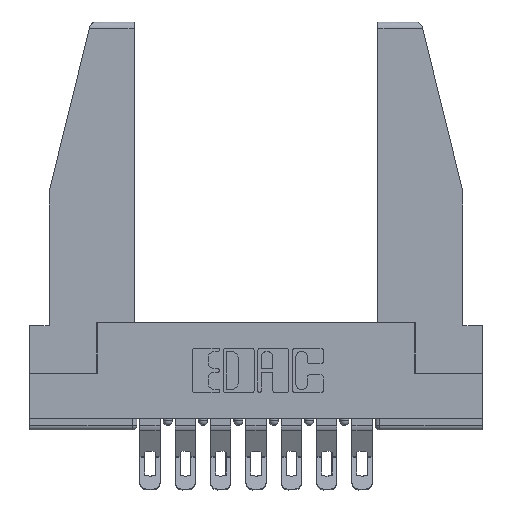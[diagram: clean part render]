
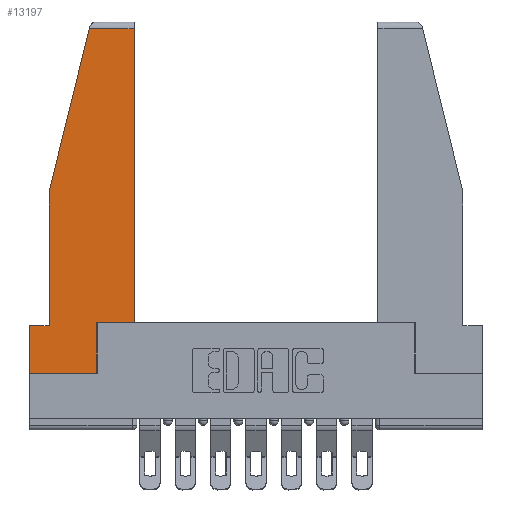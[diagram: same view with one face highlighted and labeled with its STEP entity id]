
A CAD part, top view. The second image highlights one B-rep face of the part: STEP entity #13197.
In plain terms, the highlighted planar face has unit normal (0, 0, 1).
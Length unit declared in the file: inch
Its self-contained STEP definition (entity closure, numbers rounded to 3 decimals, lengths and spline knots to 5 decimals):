
#90 = VERTEX_POINT ( 'NONE', #495 ) ;
#117 = CARTESIAN_POINT ( 'NONE',  ( 0.086, 0.21, 0. ) ) ;
#325 = LINE ( 'NONE', #3770, #1312 ) ;
#362 = CARTESIAN_POINT ( 'NONE',  ( 0.297, 0.223, 0. ) ) ;
#422 = EDGE_LOOP ( 'NONE', ( #8226, #6201, #9857, #6817, #12835, #5437, #7567, #5539, #12540 ) ) ;
#495 = CARTESIAN_POINT ( 'NONE',  ( 0., 0.21, 0. ) ) ;
#520 = CARTESIAN_POINT ( 'NONE',  ( 0., 0.21, 0. ) ) ;
#889 = VECTOR ( 'NONE', #11990, 39.37008 ) ;
#1147 = CARTESIAN_POINT ( 'NONE',  ( 0., 1.52, 0. ) ) ;
#1178 = CARTESIAN_POINT ( 'NONE',  ( 0.297, 0.223, 0. ) ) ;
#1312 = VECTOR ( 'NONE', #1547, 39.37008 ) ;
#1526 = VERTEX_POINT ( 'NONE', #117 ) ;
#1547 = DIRECTION ( 'NONE',  ( -0.239, -0.971, 0. ) ) ;
#1592 = CARTESIAN_POINT ( 'NONE',  ( 0., 0., 0. ) ) ;
#1813 = VECTOR ( 'NONE', #8463, 39.37008 ) ;
#1861 = CARTESIAN_POINT ( 'NONE',  ( 0., 0., 0. ) ) ;
#1999 = EDGE_CURVE ( 'NONE', #7309, #3363, #325, .T. ) ;
#2274 = CARTESIAN_POINT ( 'NONE',  ( 0.086, 0.8, 0. ) ) ;
#2458 = DIRECTION ( 'NONE',  ( 0., 1., 0. ) ) ;
#2644 = DIRECTION ( 'NONE',  ( 0., -1., 0. ) ) ;
#3349 = LINE ( 'NONE', #362, #6146 ) ;
#3363 = VERTEX_POINT ( 'NONE', #2274 ) ;
#3601 = CARTESIAN_POINT ( 'NONE',  ( 0.461, 0.223, 0. ) ) ;
#3629 = DIRECTION ( 'NONE',  ( 1., 0., 0. ) ) ;
#3770 = CARTESIAN_POINT ( 'NONE',  ( 0.271, 1.55, 0. ) ) ;
#3866 = VECTOR ( 'NONE', #2458, 39.37008 ) ;
#3946 = LINE ( 'NONE', #1147, #1813 ) ;
#4187 = EDGE_CURVE ( 'NONE', #5553, #9948, #3349, .T. ) ;
#4258 = DIRECTION ( 'NONE',  ( 1., 0., 0. ) ) ;
#4366 = CARTESIAN_POINT ( 'NONE',  ( 0.2636, 1.52, 0. ) ) ;
#4369 = CARTESIAN_POINT ( 'NONE',  ( 0.461, 0.223, 0. ) ) ;
#4576 = CARTESIAN_POINT ( 'NONE',  ( 0.461, 1.52, 0. ) ) ;
#4692 = DIRECTION ( 'NONE',  ( -1., 0., 0. ) ) ;
#4733 = CARTESIAN_POINT ( 'NONE',  ( 0., 0.21, 0. ) ) ;
#4796 = CARTESIAN_POINT ( 'NONE',  ( 0., 0., 0. ) ) ;
#4807 = VERTEX_POINT ( 'NONE', #4576 ) ;
#4855 = CARTESIAN_POINT ( 'NONE',  ( 0.297, 0., 0. ) ) ;
#5427 = AXIS2_PLACEMENT_3D ( 'NONE', #1861, #13531, #4258 ) ;
#5437 = ORIENTED_EDGE ( 'NONE', *, *, #6322, .T. ) ;
#5539 = ORIENTED_EDGE ( 'NONE', *, *, #10140, .T. ) ;
#5553 = VERTEX_POINT ( 'NONE', #1178 ) ;
#5555 = CARTESIAN_POINT ( 'NONE',  ( 0.297, 0., 0. ) ) ;
#5846 = LINE ( 'NONE', #3601, #3866 ) ;
#6127 = LINE ( 'NONE', #7533, #7587 ) ;
#6146 = VECTOR ( 'NONE', #3629, 39.37008 ) ;
#6201 = ORIENTED_EDGE ( 'NONE', *, *, #6682, .T. ) ;
#6322 = EDGE_CURVE ( 'NONE', #90, #11217, #8530, .T. ) ;
#6682 = EDGE_CURVE ( 'NONE', #4807, #7309, #3946, .T. ) ;
#6817 = ORIENTED_EDGE ( 'NONE', *, *, #12252, .T. ) ;
#7309 = VERTEX_POINT ( 'NONE', #4366 ) ;
#7518 = VECTOR ( 'NONE', #4692, 39.37008 ) ;
#7533 = CARTESIAN_POINT ( 'NONE',  ( 0.086, 0.8, 0. ) ) ;
#7567 = ORIENTED_EDGE ( 'NONE', *, *, #10977, .T. ) ;
#7587 = VECTOR ( 'NONE', #8563, 39.37008 ) ;
#8046 = EDGE_CURVE ( 'NONE', #1526, #90, #10918, .T. ) ;
#8186 = PLANE ( 'NONE',  #5427 ) ;
#8205 = FACE_OUTER_BOUND ( 'NONE', #422, .T. ) ;
#8226 = ORIENTED_EDGE ( 'NONE', *, *, #10840, .T. ) ;
#8463 = DIRECTION ( 'NONE',  ( -1., 0., 0. ) ) ;
#8530 = LINE ( 'NONE', #520, #13094 ) ;
#8563 = DIRECTION ( 'NONE',  ( 0., -1., 0. ) ) ;
#8775 = DIRECTION ( 'NONE',  ( 0., 1., 0. ) ) ;
#9252 = LINE ( 'NONE', #4796, #889 ) ;
#9439 = LINE ( 'NONE', #5555, #11381 ) ;
#9857 = ORIENTED_EDGE ( 'NONE', *, *, #1999, .T. ) ;
#9948 = VERTEX_POINT ( 'NONE', #4369 ) ;
#10140 = EDGE_CURVE ( 'NONE', #11886, #5553, #9439, .T. ) ;
#10840 = EDGE_CURVE ( 'NONE', #9948, #4807, #5846, .T. ) ;
#10918 = LINE ( 'NONE', #4733, #7518 ) ;
#10977 = EDGE_CURVE ( 'NONE', #11217, #11886, #9252, .T. ) ;
#11217 = VERTEX_POINT ( 'NONE', #1592 ) ;
#11381 = VECTOR ( 'NONE', #8775, 39.37008 ) ;
#11886 = VERTEX_POINT ( 'NONE', #4855 ) ;
#11990 = DIRECTION ( 'NONE',  ( 1., 0., 0. ) ) ;
#12252 = EDGE_CURVE ( 'NONE', #3363, #1526, #6127, .T. ) ;
#12540 = ORIENTED_EDGE ( 'NONE', *, *, #4187, .T. ) ;
#12835 = ORIENTED_EDGE ( 'NONE', *, *, #8046, .T. ) ;
#13094 = VECTOR ( 'NONE', #2644, 39.37008 ) ;
#13197 = ADVANCED_FACE ( 'NONE', ( #8205 ), #8186, .T. ) ;
#13531 = DIRECTION ( 'NONE',  ( 0., 0., 1. ) ) ;
